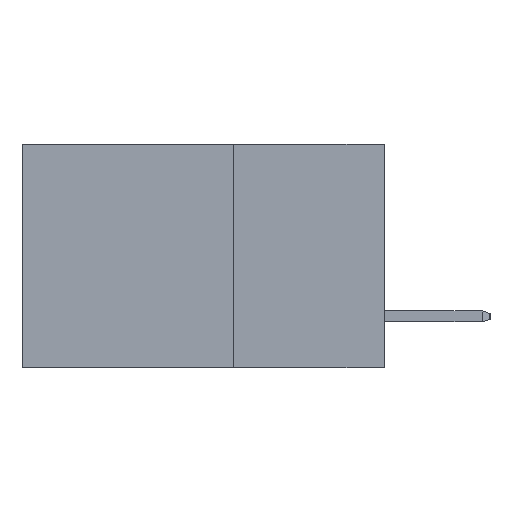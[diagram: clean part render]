
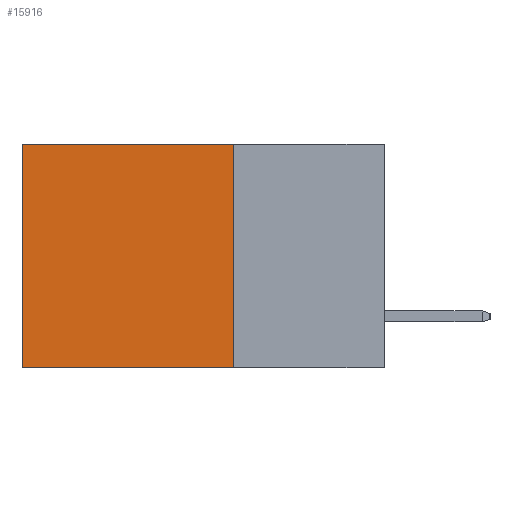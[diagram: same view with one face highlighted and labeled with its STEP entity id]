
A CAD part, left-side view. The second image highlights one B-rep face of the part: STEP entity #15916.
In plain terms, the highlighted planar face has unit normal (-1, 0, 0).
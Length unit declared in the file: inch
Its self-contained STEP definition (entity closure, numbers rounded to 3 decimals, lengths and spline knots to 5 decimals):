
#483 = VERTEX_POINT ( 'NONE', #12868 ) ;
#635 = CARTESIAN_POINT ( 'NONE',  ( 0.298, 0.6, -0.37 ) ) ;
#1205 = AXIS2_PLACEMENT_3D ( 'NONE', #10072, #15077, #7504 ) ;
#2216 = CARTESIAN_POINT ( 'NONE',  ( 0.298, 0.25, 0. ) ) ;
#2281 = DIRECTION ( 'NONE',  ( 0., 0., -1. ) ) ;
#2511 = CARTESIAN_POINT ( 'NONE',  ( 0.298, 0.25, 0. ) ) ;
#2638 = DIRECTION ( 'NONE',  ( 0., 0., -1. ) ) ;
#2726 = VERTEX_POINT ( 'NONE', #2511 ) ;
#3143 = VECTOR ( 'NONE', #2281, 39.37008 ) ;
#4257 = DIRECTION ( 'NONE',  ( 0., 1., 0. ) ) ;
#4362 = CARTESIAN_POINT ( 'NONE',  ( 0.298, 0.25, -0.37 ) ) ;
#4722 = EDGE_LOOP ( 'NONE', ( #8092, #8352, #16841, #15377 ) ) ;
#4724 = EDGE_CURVE ( 'NONE', #2726, #13691, #10834, .T. ) ;
#4971 = VERTEX_POINT ( 'NONE', #635 ) ;
#5526 = EDGE_CURVE ( 'NONE', #483, #4971, #6071, .T. ) ;
#6071 = LINE ( 'NONE', #4362, #12145 ) ;
#6129 = PLANE ( 'NONE',  #1205 ) ;
#7275 = LINE ( 'NONE', #2216, #3143 ) ;
#7457 = EDGE_CURVE ( 'NONE', #13691, #4971, #15689, .T. ) ;
#7504 = DIRECTION ( 'NONE',  ( 0., 0., -1. ) ) ;
#7596 = FACE_OUTER_BOUND ( 'NONE', #4722, .T. ) ;
#8092 = ORIENTED_EDGE ( 'NONE', *, *, #7457, .T. ) ;
#8352 = ORIENTED_EDGE ( 'NONE', *, *, #5526, .F. ) ;
#8388 = CARTESIAN_POINT ( 'NONE',  ( 0.298, 0.25, 0. ) ) ;
#8539 = DIRECTION ( 'NONE',  ( 0., 1., 0. ) ) ;
#9643 = EDGE_CURVE ( 'NONE', #2726, #483, #7275, .T. ) ;
#10072 = CARTESIAN_POINT ( 'NONE',  ( 0.298, 0.25, 0. ) ) ;
#10372 = CARTESIAN_POINT ( 'NONE',  ( 0.298, 0.6, 0. ) ) ;
#10834 = LINE ( 'NONE', #8388, #13704 ) ;
#12145 = VECTOR ( 'NONE', #4257, 39.37008 ) ;
#12341 = VECTOR ( 'NONE', #2638, 39.37008 ) ;
#12868 = CARTESIAN_POINT ( 'NONE',  ( 0.298, 0.25, -0.37 ) ) ;
#13691 = VERTEX_POINT ( 'NONE', #10372 ) ;
#13704 = VECTOR ( 'NONE', #8539, 39.37008 ) ;
#14424 = CARTESIAN_POINT ( 'NONE',  ( 0.298, 0.6, 0. ) ) ;
#15077 = DIRECTION ( 'NONE',  ( 1., 0., 0. ) ) ;
#15377 = ORIENTED_EDGE ( 'NONE', *, *, #4724, .T. ) ;
#15689 = LINE ( 'NONE', #14424, #12341 ) ;
#15916 = ADVANCED_FACE ( 'NONE', ( #7596 ), #6129, .F. ) ;
#16841 = ORIENTED_EDGE ( 'NONE', *, *, #9643, .F. ) ;
